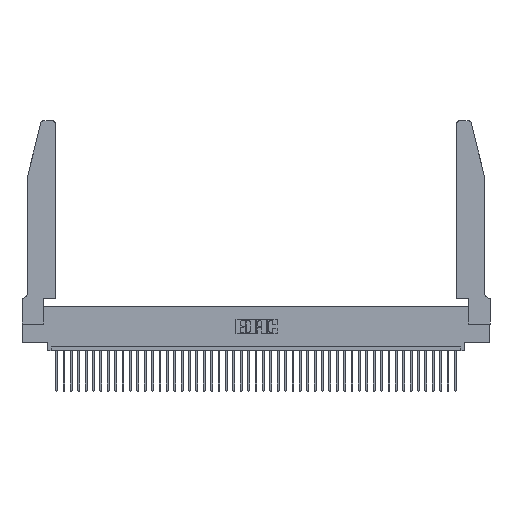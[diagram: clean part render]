
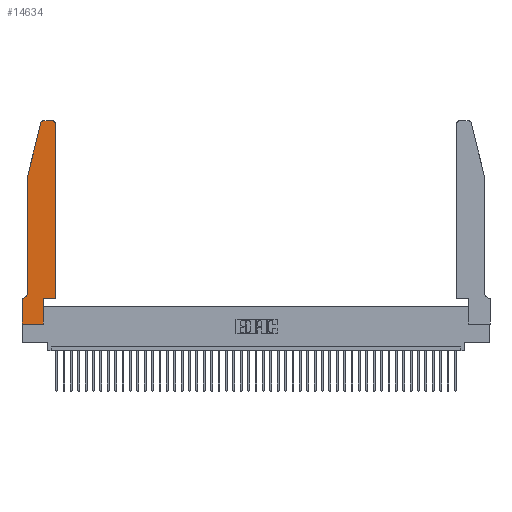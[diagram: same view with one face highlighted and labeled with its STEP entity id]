
A CAD part, top view. The second image highlights one B-rep face of the part: STEP entity #14634.
In plain terms, the highlighted planar face has unit normal (0, 0, 1).
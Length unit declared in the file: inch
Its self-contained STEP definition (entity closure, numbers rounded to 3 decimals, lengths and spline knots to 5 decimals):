
#583 = VERTEX_POINT ( 'NONE', #1024 ) ;
#781 = ORIENTED_EDGE ( 'NONE', *, *, #27925, .T. ) ;
#977 = ORIENTED_EDGE ( 'NONE', *, *, #15974, .T. ) ;
#1024 = CARTESIAN_POINT ( 'NONE',  ( 0.2865, 0.35, 0.37 ) ) ;
#1178 = LINE ( 'NONE', #23768, #23947 ) ;
#2175 = CARTESIAN_POINT ( 'NONE',  ( 0.4205, 2.72, 0.37 ) ) ;
#2832 = VECTOR ( 'NONE', #13662, 39.37008 ) ;
#2945 = LINE ( 'NONE', #39458, #14252 ) ;
#3510 = CARTESIAN_POINT ( 'NONE',  ( 0.4505, 2.72, 0.37 ) ) ;
#3554 = CARTESIAN_POINT ( 'NONE',  ( 0.0055, 0.42, 0.37 ) ) ;
#4419 = AXIS2_PLACEMENT_3D ( 'NONE', #3554, #10363, #38172 ) ;
#4718 = VERTEX_POINT ( 'NONE', #22017 ) ;
#5054 = ORIENTED_EDGE ( 'NONE', *, *, #17737, .T. ) ;
#5762 = AXIS2_PLACEMENT_3D ( 'NONE', #2175, #26365, #12590 ) ;
#5858 = DIRECTION ( 'NONE',  ( 0., -1., 0. ) ) ;
#6550 = LINE ( 'NONE', #24986, #42619 ) ;
#6557 = DIRECTION ( 'NONE',  ( 1., 0., 0. ) ) ;
#6961 = DIRECTION ( 'NONE',  ( 0., 1., 0. ) ) ;
#7345 = VERTEX_POINT ( 'NONE', #13631 ) ;
#8155 = EDGE_CURVE ( 'NONE', #27057, #9949, #2945, .T. ) ;
#8297 = DIRECTION ( 'NONE',  ( -0.239, -0.971, 0. ) ) ;
#8445 = CARTESIAN_POINT ( 'NONE',  ( 0.0755, 2., 0.37 ) ) ;
#8874 = LINE ( 'NONE', #20294, #26193 ) ;
#9174 = CARTESIAN_POINT ( 'NONE',  ( 0.0755, 2., 0.37 ) ) ;
#9800 = EDGE_CURVE ( 'NONE', #23704, #25176, #23229, .T. ) ;
#9949 = VERTEX_POINT ( 'NONE', #8445 ) ;
#10363 = DIRECTION ( 'NONE',  ( 0., 0., -1. ) ) ;
#10675 = CARTESIAN_POINT ( 'NONE',  ( 0.0755, 0.35, 0.37 ) ) ;
#11532 = DIRECTION ( 'NONE',  ( 0., 1., 0. ) ) ;
#11742 = EDGE_CURVE ( 'NONE', #25176, #35160, #19341, .T. ) ;
#12247 = CARTESIAN_POINT ( 'NONE',  ( 0.2605, 2.75, 0.37 ) ) ;
#12590 = DIRECTION ( 'NONE',  ( 1., 0., 0. ) ) ;
#12751 = ORIENTED_EDGE ( 'NONE', *, *, #18591, .T. ) ;
#13631 = CARTESIAN_POINT ( 'NONE',  ( 0.0755, 0.42, 0.37 ) ) ;
#13662 = DIRECTION ( 'NONE',  ( -1., 0., 0. ) ) ;
#14248 = PLANE ( 'NONE',  #33028 ) ;
#14252 = VECTOR ( 'NONE', #8297, 39.37008 ) ;
#14612 = ORIENTED_EDGE ( 'NONE', *, *, #43966, .T. ) ;
#14634 = ADVANCED_FACE ( 'NONE', ( #31907 ), #14248, .T. ) ;
#15782 = CARTESIAN_POINT ( 'NONE',  ( 0.284, 2.72, 0.37 ) ) ;
#15974 = EDGE_CURVE ( 'NONE', #35160, #27057, #17150, .T. ) ;
#17150 = CIRCLE ( 'NONE', #39936, 0.03 ) ;
#17737 = EDGE_CURVE ( 'NONE', #9949, #7345, #28280, .T. ) ;
#17938 = CARTESIAN_POINT ( 'NONE',  ( 0., 0.35, 0.37 ) ) ;
#18414 = CARTESIAN_POINT ( 'NONE',  ( 0.4505, 0.35, 0.37 ) ) ;
#18591 = EDGE_CURVE ( 'NONE', #25180, #4718, #40579, .T. ) ;
#19341 = LINE ( 'NONE', #12247, #39163 ) ;
#19867 = VERTEX_POINT ( 'NONE', #18414 ) ;
#20104 = VECTOR ( 'NONE', #22349, 39.37008 ) ;
#20159 = ORIENTED_EDGE ( 'NONE', *, *, #38395, .T. ) ;
#20294 = CARTESIAN_POINT ( 'NONE',  ( 0., 0., 0.37 ) ) ;
#20919 = ORIENTED_EDGE ( 'NONE', *, *, #9800, .T. ) ;
#21410 = CARTESIAN_POINT ( 'NONE',  ( 0.25487, 2.72718, 0.37 ) ) ;
#22017 = CARTESIAN_POINT ( 'NONE',  ( 0., 0.35, 0.37 ) ) ;
#22349 = DIRECTION ( 'NONE',  ( 0., -1., 0. ) ) ;
#22487 = ORIENTED_EDGE ( 'NONE', *, *, #27628, .T. ) ;
#23201 = DIRECTION ( 'NONE',  ( 1., 0., 0. ) ) ;
#23229 = CIRCLE ( 'NONE', #5762, 0.03 ) ;
#23704 = VERTEX_POINT ( 'NONE', #3510 ) ;
#23768 = CARTESIAN_POINT ( 'NONE',  ( 0.4505, 0.35, 0.37 ) ) ;
#23870 = VECTOR ( 'NONE', #11532, 39.37008 ) ;
#23947 = VECTOR ( 'NONE', #6961, 39.37008 ) ;
#24733 = ORIENTED_EDGE ( 'NONE', *, *, #11742, .T. ) ;
#24986 = CARTESIAN_POINT ( 'NONE',  ( 0.4505, 0.35, 0.37 ) ) ;
#25176 = VERTEX_POINT ( 'NONE', #35840 ) ;
#25180 = VERTEX_POINT ( 'NONE', #39298 ) ;
#26193 = VECTOR ( 'NONE', #6557, 39.37008 ) ;
#26365 = DIRECTION ( 'NONE',  ( 0., 0., 1. ) ) ;
#26638 = ORIENTED_EDGE ( 'NONE', *, *, #8155, .T. ) ;
#27057 = VERTEX_POINT ( 'NONE', #21410 ) ;
#27628 = EDGE_CURVE ( 'NONE', #583, #19867, #6550, .T. ) ;
#27925 = EDGE_CURVE ( 'NONE', #41123, #583, #32961, .T. ) ;
#28280 = LINE ( 'NONE', #9174, #43782 ) ;
#28578 = CARTESIAN_POINT ( 'NONE',  ( 0.2865, 0.35, 0.37 ) ) ;
#28990 = DIRECTION ( 'NONE',  ( -1., 0., 0. ) ) ;
#29787 = DIRECTION ( 'NONE',  ( 0., 0., 1. ) ) ;
#30639 = EDGE_CURVE ( 'NONE', #34516, #41123, #8874, .T. ) ;
#31441 = EDGE_CURVE ( 'NONE', #4718, #34516, #37835, .T. ) ;
#31891 = DIRECTION ( 'NONE',  ( 1., 0., 0. ) ) ;
#31907 = FACE_OUTER_BOUND ( 'NONE', #41653, .T. ) ;
#31993 = ORIENTED_EDGE ( 'NONE', *, *, #30639, .T. ) ;
#32961 = LINE ( 'NONE', #28578, #23870 ) ;
#33028 = AXIS2_PLACEMENT_3D ( 'NONE', #17938, #34742, #31891 ) ;
#33232 = CIRCLE ( 'NONE', #4419, 0.07 ) ;
#34495 = CARTESIAN_POINT ( 'NONE',  ( 0.2865, 0., 0.37 ) ) ;
#34516 = VERTEX_POINT ( 'NONE', #44051 ) ;
#34742 = DIRECTION ( 'NONE',  ( 0., 0., 1. ) ) ;
#35160 = VERTEX_POINT ( 'NONE', #41211 ) ;
#35840 = CARTESIAN_POINT ( 'NONE',  ( 0.4205, 2.75, 0.37 ) ) ;
#37835 = LINE ( 'NONE', #43294, #20104 ) ;
#38172 = DIRECTION ( 'NONE',  ( -1., 0., 0. ) ) ;
#38395 = EDGE_CURVE ( 'NONE', #7345, #25180, #33232, .T. ) ;
#38784 = DIRECTION ( 'NONE',  ( 1., 0., 0. ) ) ;
#39163 = VECTOR ( 'NONE', #28990, 39.37008 ) ;
#39298 = CARTESIAN_POINT ( 'NONE',  ( 0.0055, 0.35, 0.37 ) ) ;
#39458 = CARTESIAN_POINT ( 'NONE',  ( 0.0755, 2., 0.37 ) ) ;
#39936 = AXIS2_PLACEMENT_3D ( 'NONE', #15782, #29787, #23201 ) ;
#40579 = LINE ( 'NONE', #10675, #2832 ) ;
#41123 = VERTEX_POINT ( 'NONE', #34495 ) ;
#41211 = CARTESIAN_POINT ( 'NONE',  ( 0.284, 2.75, 0.37 ) ) ;
#41270 = ORIENTED_EDGE ( 'NONE', *, *, #31441, .T. ) ;
#41653 = EDGE_LOOP ( 'NONE', ( #24733, #977, #26638, #5054, #20159, #12751, #41270, #31993, #781, #22487, #14612, #20919 ) ) ;
#42619 = VECTOR ( 'NONE', #38784, 39.37008 ) ;
#43294 = CARTESIAN_POINT ( 'NONE',  ( 0., 0., 0.37 ) ) ;
#43782 = VECTOR ( 'NONE', #5858, 39.37008 ) ;
#43966 = EDGE_CURVE ( 'NONE', #19867, #23704, #1178, .T. ) ;
#44051 = CARTESIAN_POINT ( 'NONE',  ( 0., 0., 0.37 ) ) ;
